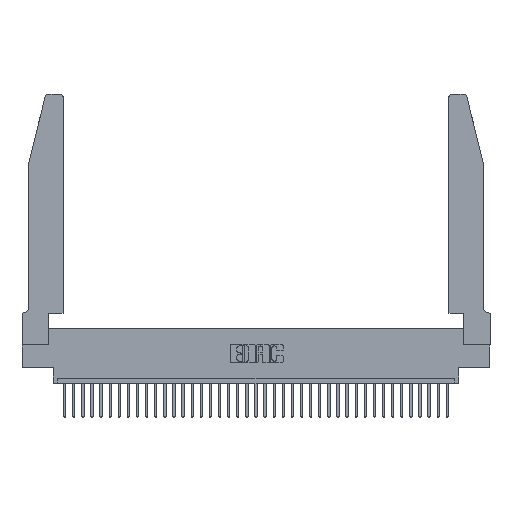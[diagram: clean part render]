
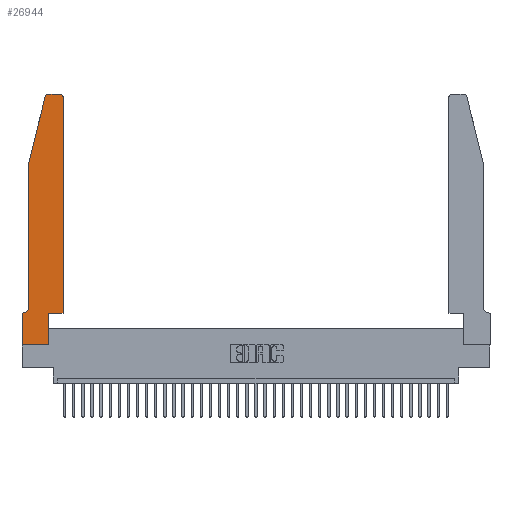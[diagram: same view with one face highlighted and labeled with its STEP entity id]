
A CAD part, top view. The second image highlights one B-rep face of the part: STEP entity #26944.
In plain terms, the highlighted planar face has unit normal (0, 0, 1).
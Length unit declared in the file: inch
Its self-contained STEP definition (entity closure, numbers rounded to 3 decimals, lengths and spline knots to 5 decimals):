
#151 = VERTEX_POINT ( 'NONE', #18701 ) ;
#345 = VERTEX_POINT ( 'NONE', #1554 ) ;
#399 = VERTEX_POINT ( 'NONE', #11406 ) ;
#688 = FACE_OUTER_BOUND ( 'NONE', #10031, .T. ) ;
#797 = VECTOR ( 'NONE', #6850, 39.37008 ) ;
#841 = DIRECTION ( 'NONE',  ( 1., 0., 0. ) ) ;
#1236 = VERTEX_POINT ( 'NONE', #12199 ) ;
#1554 = CARTESIAN_POINT ( 'NONE',  ( 0., 0.35, 0.37 ) ) ;
#2015 = VERTEX_POINT ( 'NONE', #7822 ) ;
#2950 = DIRECTION ( 'NONE',  ( 0., 1., 0. ) ) ;
#3734 = ORIENTED_EDGE ( 'NONE', *, *, #13492, .T. ) ;
#3736 = CARTESIAN_POINT ( 'NONE',  ( 0., 0.35, 0.37 ) ) ;
#3789 = CARTESIAN_POINT ( 'NONE',  ( 0.0055, 0.42, 0.37 ) ) ;
#5211 = VERTEX_POINT ( 'NONE', #9860 ) ;
#5769 = AXIS2_PLACEMENT_3D ( 'NONE', #3736, #12719, #841 ) ;
#5858 = VERTEX_POINT ( 'NONE', #33840 ) ;
#6530 = AXIS2_PLACEMENT_3D ( 'NONE', #14961, #20705, #23086 ) ;
#6541 = CIRCLE ( 'NONE', #22875, 0.03 ) ;
#6683 = DIRECTION ( 'NONE',  ( 0., 0., -1. ) ) ;
#6850 = DIRECTION ( 'NONE',  ( 0., -1., 0. ) ) ;
#6887 = ORIENTED_EDGE ( 'NONE', *, *, #8034, .T. ) ;
#7822 = CARTESIAN_POINT ( 'NONE',  ( 0., 0., 0.37 ) ) ;
#8034 = EDGE_CURVE ( 'NONE', #5211, #24083, #21026, .T. ) ;
#8294 = VERTEX_POINT ( 'NONE', #13168 ) ;
#8883 = AXIS2_PLACEMENT_3D ( 'NONE', #3789, #6683, #26714 ) ;
#9326 = ORIENTED_EDGE ( 'NONE', *, *, #12823, .T. ) ;
#9465 = CIRCLE ( 'NONE', #6530, 0.03 ) ;
#9559 = CARTESIAN_POINT ( 'NONE',  ( 0.4505, 0.35, 0.37 ) ) ;
#9860 = CARTESIAN_POINT ( 'NONE',  ( 0.4205, 2.75, 0.37 ) ) ;
#10031 = EDGE_LOOP ( 'NONE', ( #6887, #16731, #26143, #13108, #9326, #3734, #17663, #16760, #18525, #34047, #17118, #15551 ) ) ;
#10066 = CARTESIAN_POINT ( 'NONE',  ( 0.0755, 2., 0.37 ) ) ;
#11074 = VECTOR ( 'NONE', #28750, 39.37008 ) ;
#11406 = CARTESIAN_POINT ( 'NONE',  ( 0.0755, 0.42, 0.37 ) ) ;
#11440 = DIRECTION ( 'NONE',  ( 1., 0., 0. ) ) ;
#11876 = LINE ( 'NONE', #22933, #33514 ) ;
#12199 = CARTESIAN_POINT ( 'NONE',  ( 0.25487, 2.72718, 0.37 ) ) ;
#12650 = VECTOR ( 'NONE', #21887, 39.37008 ) ;
#12719 = DIRECTION ( 'NONE',  ( 0., 0., 1. ) ) ;
#12823 = EDGE_CURVE ( 'NONE', #399, #33991, #16756, .T. ) ;
#13106 = EDGE_CURVE ( 'NONE', #1236, #15239, #23364, .T. ) ;
#13108 = ORIENTED_EDGE ( 'NONE', *, *, #32247, .T. ) ;
#13168 = CARTESIAN_POINT ( 'NONE',  ( 0.2865, 0., 0.37 ) ) ;
#13492 = EDGE_CURVE ( 'NONE', #33991, #345, #20189, .T. ) ;
#13785 = CARTESIAN_POINT ( 'NONE',  ( 0.0755, 0.35, 0.37 ) ) ;
#14961 = CARTESIAN_POINT ( 'NONE',  ( 0.4205, 2.72, 0.37 ) ) ;
#15239 = VERTEX_POINT ( 'NONE', #10066 ) ;
#15332 = CARTESIAN_POINT ( 'NONE',  ( 0., 0., 0.37 ) ) ;
#15551 = ORIENTED_EDGE ( 'NONE', *, *, #29394, .T. ) ;
#16731 = ORIENTED_EDGE ( 'NONE', *, *, #22147, .T. ) ;
#16756 = CIRCLE ( 'NONE', #8883, 0.07 ) ;
#16760 = ORIENTED_EDGE ( 'NONE', *, *, #24100, .T. ) ;
#17043 = VECTOR ( 'NONE', #18954, 39.37008 ) ;
#17118 = ORIENTED_EDGE ( 'NONE', *, *, #33069, .T. ) ;
#17663 = ORIENTED_EDGE ( 'NONE', *, *, #25304, .T. ) ;
#17780 = DIRECTION ( 'NONE',  ( 1., 0., 0. ) ) ;
#18525 = ORIENTED_EDGE ( 'NONE', *, *, #28559, .T. ) ;
#18559 = CARTESIAN_POINT ( 'NONE',  ( 0.284, 2.72, 0.37 ) ) ;
#18701 = CARTESIAN_POINT ( 'NONE',  ( 0.4505, 0.35, 0.37 ) ) ;
#18717 = DIRECTION ( 'NONE',  ( 0., 0., 1. ) ) ;
#18954 = DIRECTION ( 'NONE',  ( -1., 0., 0. ) ) ;
#19074 = CARTESIAN_POINT ( 'NONE',  ( 0.2605, 2.75, 0.37 ) ) ;
#19658 = LINE ( 'NONE', #33914, #33645 ) ;
#19932 = LINE ( 'NONE', #9559, #33899 ) ;
#20189 = LINE ( 'NONE', #13785, #31920 ) ;
#20232 = LINE ( 'NONE', #27834, #12650 ) ;
#20705 = DIRECTION ( 'NONE',  ( 0., 0., 1. ) ) ;
#20850 = LINE ( 'NONE', #34497, #11074 ) ;
#21026 = LINE ( 'NONE', #19074, #17043 ) ;
#21454 = CARTESIAN_POINT ( 'NONE',  ( 0.284, 2.75, 0.37 ) ) ;
#21692 = VERTEX_POINT ( 'NONE', #29909 ) ;
#21887 = DIRECTION ( 'NONE',  ( 0., 1., 0. ) ) ;
#22147 = EDGE_CURVE ( 'NONE', #24083, #1236, #6541, .T. ) ;
#22875 = AXIS2_PLACEMENT_3D ( 'NONE', #18559, #18717, #17780 ) ;
#22933 = CARTESIAN_POINT ( 'NONE',  ( 0.4505, 0.35, 0.37 ) ) ;
#23086 = DIRECTION ( 'NONE',  ( 1., 0., 0. ) ) ;
#23364 = LINE ( 'NONE', #32592, #27500 ) ;
#24083 = VERTEX_POINT ( 'NONE', #21454 ) ;
#24100 = EDGE_CURVE ( 'NONE', #2015, #8294, #19658, .T. ) ;
#24135 = PLANE ( 'NONE',  #5769 ) ;
#25304 = EDGE_CURVE ( 'NONE', #345, #2015, #29514, .T. ) ;
#26143 = ORIENTED_EDGE ( 'NONE', *, *, #13106, .T. ) ;
#26714 = DIRECTION ( 'NONE',  ( -1., 0., 0. ) ) ;
#26944 = ADVANCED_FACE ( 'NONE', ( #688 ), #24135, .T. ) ;
#27500 = VECTOR ( 'NONE', #32322, 39.37008 ) ;
#27834 = CARTESIAN_POINT ( 'NONE',  ( 0.2865, 0.35, 0.37 ) ) ;
#28241 = DIRECTION ( 'NONE',  ( -1., 0., 0. ) ) ;
#28559 = EDGE_CURVE ( 'NONE', #8294, #5858, #20232, .T. ) ;
#28750 = DIRECTION ( 'NONE',  ( 0., -1., 0. ) ) ;
#29394 = EDGE_CURVE ( 'NONE', #21692, #5211, #9465, .T. ) ;
#29514 = LINE ( 'NONE', #15332, #797 ) ;
#29909 = CARTESIAN_POINT ( 'NONE',  ( 0.4505, 2.72, 0.37 ) ) ;
#31920 = VECTOR ( 'NONE', #28241, 39.37008 ) ;
#32247 = EDGE_CURVE ( 'NONE', #15239, #399, #20850, .T. ) ;
#32322 = DIRECTION ( 'NONE',  ( -0.239, -0.971, 0. ) ) ;
#32592 = CARTESIAN_POINT ( 'NONE',  ( 0.0755, 2., 0.37 ) ) ;
#33069 = EDGE_CURVE ( 'NONE', #151, #21692, #11876, .T. ) ;
#33347 = EDGE_CURVE ( 'NONE', #5858, #151, #19932, .T. ) ;
#33514 = VECTOR ( 'NONE', #2950, 39.37008 ) ;
#33645 = VECTOR ( 'NONE', #11440, 39.37008 ) ;
#33840 = CARTESIAN_POINT ( 'NONE',  ( 0.2865, 0.35, 0.37 ) ) ;
#33899 = VECTOR ( 'NONE', #35267, 39.37008 ) ;
#33914 = CARTESIAN_POINT ( 'NONE',  ( 0., 0., 0.37 ) ) ;
#33991 = VERTEX_POINT ( 'NONE', #34829 ) ;
#34047 = ORIENTED_EDGE ( 'NONE', *, *, #33347, .T. ) ;
#34497 = CARTESIAN_POINT ( 'NONE',  ( 0.0755, 2., 0.37 ) ) ;
#34829 = CARTESIAN_POINT ( 'NONE',  ( 0.0055, 0.35, 0.37 ) ) ;
#35267 = DIRECTION ( 'NONE',  ( 1., 0., 0. ) ) ;
